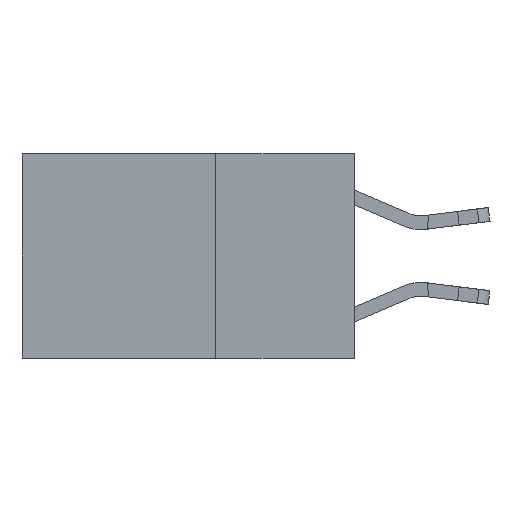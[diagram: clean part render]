
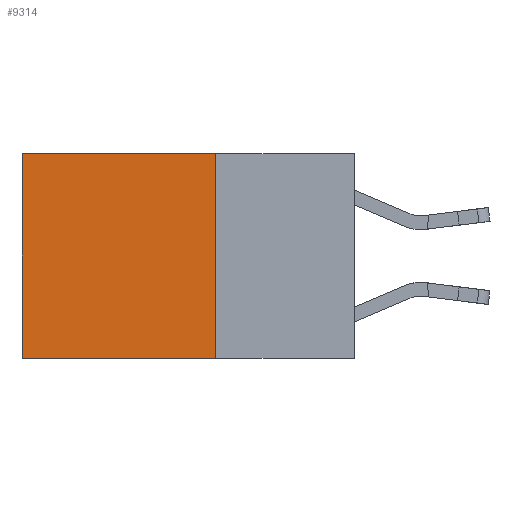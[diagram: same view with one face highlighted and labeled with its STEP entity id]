
A CAD part, left-side view. The second image highlights one B-rep face of the part: STEP entity #9314.
In plain terms, the highlighted planar face has unit normal (-1, 0, 0).
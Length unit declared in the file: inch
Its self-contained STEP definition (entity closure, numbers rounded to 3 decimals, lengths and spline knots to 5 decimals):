
#352 = EDGE_LOOP ( 'NONE', ( #12292, #6235, #9503, #12660 ) ) ;
#887 = EDGE_CURVE ( 'NONE', #9537, #12223, #4174, .T. ) ;
#1735 = CARTESIAN_POINT ( 'NONE',  ( 0.2625, 0.25, 0. ) ) ;
#2260 = CARTESIAN_POINT ( 'NONE',  ( 0.2625, 0.25, -0.37 ) ) ;
#2516 = FACE_OUTER_BOUND ( 'NONE', #352, .T. ) ;
#2722 = CARTESIAN_POINT ( 'NONE',  ( 0.2625, 0.25, -0.37 ) ) ;
#2910 = DIRECTION ( 'NONE',  ( 0., 0., -1. ) ) ;
#3581 = CARTESIAN_POINT ( 'NONE',  ( 0.2625, 0.6, 0. ) ) ;
#3614 = CARTESIAN_POINT ( 'NONE',  ( 0.2625, 0.25, 0. ) ) ;
#3855 = DIRECTION ( 'NONE',  ( 0., 1., 0. ) ) ;
#4101 = DIRECTION ( 'NONE',  ( 0., 1., 0. ) ) ;
#4174 = LINE ( 'NONE', #5136, #10196 ) ;
#4238 = CARTESIAN_POINT ( 'NONE',  ( 0.2625, 0.6, 0. ) ) ;
#4669 = VERTEX_POINT ( 'NONE', #2260 ) ;
#5136 = CARTESIAN_POINT ( 'NONE',  ( 0.2625, 0.25, 0. ) ) ;
#5170 = LINE ( 'NONE', #14225, #5547 ) ;
#5547 = VECTOR ( 'NONE', #11931, 39.37008 ) ;
#5910 = DIRECTION ( 'NONE',  ( 0., 0., -1. ) ) ;
#6235 = ORIENTED_EDGE ( 'NONE', *, *, #10545, .F. ) ;
#6246 = VECTOR ( 'NONE', #3855, 39.37008 ) ;
#7497 = PLANE ( 'NONE',  #15208 ) ;
#8205 = CARTESIAN_POINT ( 'NONE',  ( 0.2625, 0.6, -0.37 ) ) ;
#9314 = ADVANCED_FACE ( 'NONE', ( #2516 ), #7497, .F. ) ;
#9503 = ORIENTED_EDGE ( 'NONE', *, *, #10022, .F. ) ;
#9537 = VERTEX_POINT ( 'NONE', #3614 ) ;
#10022 = EDGE_CURVE ( 'NONE', #9537, #4669, #5170, .T. ) ;
#10036 = DIRECTION ( 'NONE',  ( 1., 0., 0. ) ) ;
#10196 = VECTOR ( 'NONE', #4101, 39.37008 ) ;
#10444 = EDGE_CURVE ( 'NONE', #12223, #11987, #14774, .T. ) ;
#10545 = EDGE_CURVE ( 'NONE', #4669, #11987, #12669, .T. ) ;
#11745 = VECTOR ( 'NONE', #5910, 39.37008 ) ;
#11931 = DIRECTION ( 'NONE',  ( 0., 0., -1. ) ) ;
#11987 = VERTEX_POINT ( 'NONE', #8205 ) ;
#12223 = VERTEX_POINT ( 'NONE', #4238 ) ;
#12292 = ORIENTED_EDGE ( 'NONE', *, *, #10444, .T. ) ;
#12660 = ORIENTED_EDGE ( 'NONE', *, *, #887, .T. ) ;
#12669 = LINE ( 'NONE', #2722, #6246 ) ;
#14225 = CARTESIAN_POINT ( 'NONE',  ( 0.2625, 0.25, 0. ) ) ;
#14774 = LINE ( 'NONE', #3581, #11745 ) ;
#15208 = AXIS2_PLACEMENT_3D ( 'NONE', #1735, #10036, #2910 ) ;
